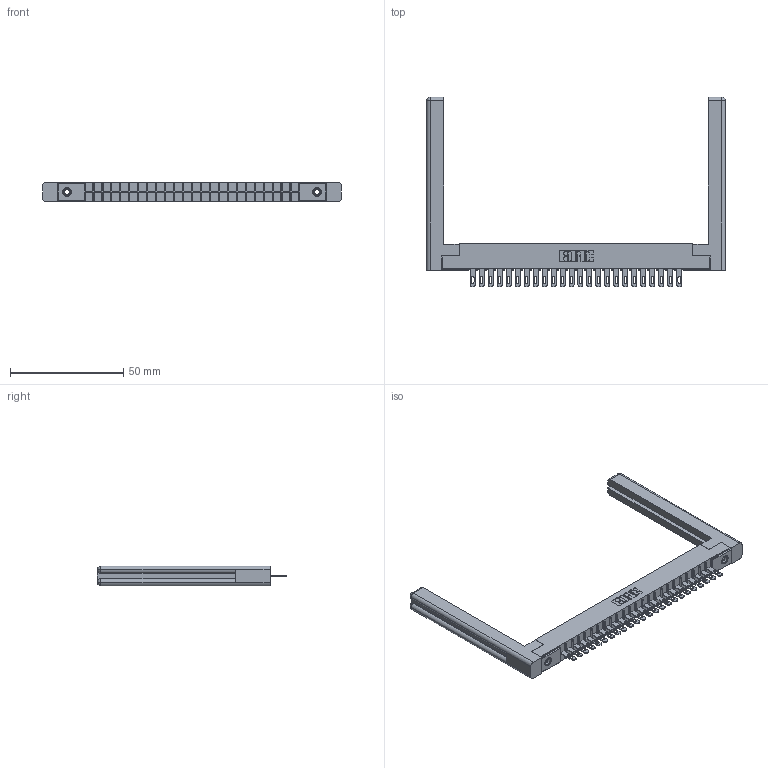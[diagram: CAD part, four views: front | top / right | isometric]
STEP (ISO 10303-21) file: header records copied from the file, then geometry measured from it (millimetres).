
FILE_DESCRIPTION (( 'STEP AP203' ), '1' );
FILE_NAME ('316-024-400-158.STEP', '2020-09-22T21:21:35', ( '' ), ( '' ), 'SwSTEP 2.0', 'SolidWorks 2020', '' );
FILE_SCHEMA (( 'CONFIG_CONTROL_DESIGN' ));
Length unit declared in the file: inch
Products named in the file (5): 306 Part_.156 Dia; 307-220-058; 345-250-001_345-250-001-102; 316-024-400-158; 306-290-001_100
Assembly tree (29 placements, depth 2):
  316-024-400-158
    306 Part_.156 Dia
    306-290-001_100  x24
    345-250-001_345-250-001-102  x2
    307-220-058  x2
Bounding box: 131.72 x 83.52 x 8.71 mm (x, y, z)
Volume: 16744.9 mm3; surface area: 19179.1 mm2
Topology: 29 solids, 29 shells, 2082 faces, 5830 edges, 3744 vertices
Faces by surface type: plane 1352, cylinder 610, sphere 96, cone 12, torus 12
Entity records: 27510 total; most frequent: CARTESIAN_POINT 4626, ORIENTED_EDGE 4526, DIRECTION 4519, EDGE_CURVE 2263, VECTOR 1753, LINE 1753, VERTEX_POINT 1436, AXIS2_PLACEMENT_3D 1383
